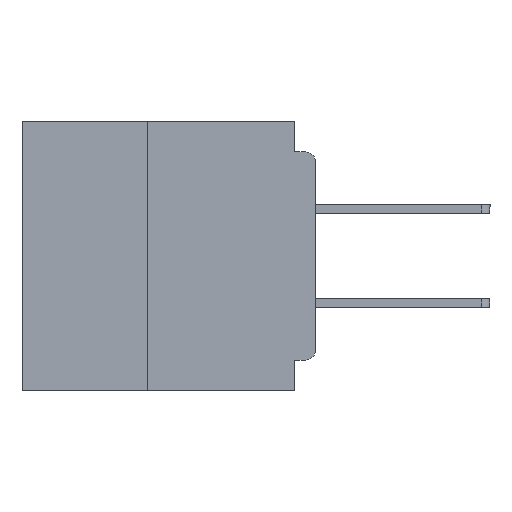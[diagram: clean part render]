
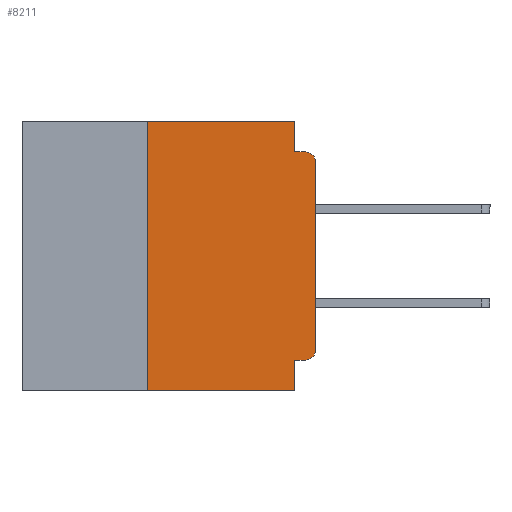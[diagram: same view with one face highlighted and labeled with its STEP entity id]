
A CAD part, left-side view. The second image highlights one B-rep face of the part: STEP entity #8211.
In plain terms, the highlighted planar face has unit normal (-1, 0, 0).
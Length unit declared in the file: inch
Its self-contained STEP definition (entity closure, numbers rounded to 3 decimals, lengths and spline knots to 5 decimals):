
#1073 = CARTESIAN_POINT ( 'NONE',  ( 0., 0., -0.34 ) ) ;
#1790 = CIRCLE ( 'NONE', #19528, 0.015 ) ;
#2159 = EDGE_CURVE ( 'NONE', #34190, #41145, #24736, .T. ) ;
#2250 = DIRECTION ( 'NONE',  ( 1., 0., 0. ) ) ;
#2364 = DIRECTION ( 'NONE',  ( 0., 0., -1. ) ) ;
#2720 = DIRECTION ( 'NONE',  ( 0., -1., 0. ) ) ;
#3563 = ORIENTED_EDGE ( 'NONE', *, *, #8190, .F. ) ;
#3602 = VERTEX_POINT ( 'NONE', #1073 ) ;
#4623 = CARTESIAN_POINT ( 'NONE',  ( 0., 0.015, -0.355 ) ) ;
#5570 = EDGE_CURVE ( 'NONE', #44614, #32273, #44536, .T. ) ;
#5735 = VECTOR ( 'NONE', #9948, 39.37008 ) ;
#6171 = CARTESIAN_POINT ( 'NONE',  ( 0., 0.437, 0. ) ) ;
#7149 = DIRECTION ( 'NONE',  ( 0., -1., 0. ) ) ;
#7772 = CARTESIAN_POINT ( 'NONE',  ( 0., 0., -0.355 ) ) ;
#8100 = EDGE_LOOP ( 'NONE', ( #29701, #22460, #29448, #16338, #37765, #3563, #18089, #26613, #38878, #15300 ) ) ;
#8190 = EDGE_CURVE ( 'NONE', #44614, #34190, #16019, .T. ) ;
#8211 = ADVANCED_FACE ( 'NONE', ( #45442 ), #40736, .F. ) ;
#9084 = VECTOR ( 'NONE', #38443, 39.37008 ) ;
#9948 = DIRECTION ( 'NONE',  ( 0., 0., 1. ) ) ;
#10064 = LINE ( 'NONE', #24833, #19144 ) ;
#10796 = EDGE_CURVE ( 'NONE', #41145, #42122, #39702, .T. ) ;
#10798 = AXIS2_PLACEMENT_3D ( 'NONE', #48417, #25735, #2364 ) ;
#11180 = DIRECTION ( 'NONE',  ( 0., 0., -1. ) ) ;
#11835 = VERTEX_POINT ( 'NONE', #25370 ) ;
#13703 = DIRECTION ( 'NONE',  ( 0., -1., 0. ) ) ;
#14224 = LINE ( 'NONE', #48257, #25846 ) ;
#14352 = VECTOR ( 'NONE', #2720, 39.37008 ) ;
#15084 = VECTOR ( 'NONE', #13703, 39.37008 ) ;
#15140 = CIRCLE ( 'NONE', #10798, 0.015 ) ;
#15300 = ORIENTED_EDGE ( 'NONE', *, *, #25182, .T. ) ;
#16019 = LINE ( 'NONE', #17402, #5735 ) ;
#16310 = EDGE_CURVE ( 'NONE', #42122, #11835, #26141, .T. ) ;
#16338 = ORIENTED_EDGE ( 'NONE', *, *, #10796, .F. ) ;
#17402 = CARTESIAN_POINT ( 'NONE',  ( 0., 0.25, -0.4 ) ) ;
#17687 = CARTESIAN_POINT ( 'NONE',  ( 0., 0.031, -0.045 ) ) ;
#18089 = ORIENTED_EDGE ( 'NONE', *, *, #5570, .T. ) ;
#19144 = VECTOR ( 'NONE', #21056, 39.37008 ) ;
#19262 = VECTOR ( 'NONE', #11180, 39.37008 ) ;
#19528 = AXIS2_PLACEMENT_3D ( 'NONE', #46022, #23209, #49741 ) ;
#21056 = DIRECTION ( 'NONE',  ( 0., 0., -1. ) ) ;
#21439 = VERTEX_POINT ( 'NONE', #39050 ) ;
#21489 = VERTEX_POINT ( 'NONE', #4623 ) ;
#22460 = ORIENTED_EDGE ( 'NONE', *, *, #35414, .T. ) ;
#22582 = CARTESIAN_POINT ( 'NONE',  ( 0., 0.25, -0.4 ) ) ;
#22644 = CARTESIAN_POINT ( 'NONE',  ( 0., 0., -0.06 ) ) ;
#23209 = DIRECTION ( 'NONE',  ( -1., 0., 0. ) ) ;
#24341 = CARTESIAN_POINT ( 'NONE',  ( 0., 0.031, -0.4 ) ) ;
#24736 = LINE ( 'NONE', #6171, #14352 ) ;
#24833 = CARTESIAN_POINT ( 'NONE',  ( 0., 0.031, -0.4 ) ) ;
#25182 = EDGE_CURVE ( 'NONE', #21489, #3602, #15140, .T. ) ;
#25370 = CARTESIAN_POINT ( 'NONE',  ( 0., 0.015, -0.045 ) ) ;
#25563 = DIRECTION ( 'NONE',  ( 0., 0., 1. ) ) ;
#25612 = CARTESIAN_POINT ( 'NONE',  ( 0., 0.437, 0. ) ) ;
#25735 = DIRECTION ( 'NONE',  ( -1., 0., 0. ) ) ;
#25846 = VECTOR ( 'NONE', #25563, 39.37008 ) ;
#26141 = LINE ( 'NONE', #38014, #45145 ) ;
#26613 = ORIENTED_EDGE ( 'NONE', *, *, #42640, .F. ) ;
#27244 = CARTESIAN_POINT ( 'NONE',  ( 0., 0.25, 0. ) ) ;
#29448 = ORIENTED_EDGE ( 'NONE', *, *, #16310, .F. ) ;
#29449 = DIRECTION ( 'NONE',  ( 0., 0., -1. ) ) ;
#29701 = ORIENTED_EDGE ( 'NONE', *, *, #39536, .T. ) ;
#30173 = VERTEX_POINT ( 'NONE', #22644 ) ;
#32273 = VERTEX_POINT ( 'NONE', #24341 ) ;
#34190 = VERTEX_POINT ( 'NONE', #27244 ) ;
#34305 = CARTESIAN_POINT ( 'NONE',  ( 0., 0.031, 0. ) ) ;
#35414 = EDGE_CURVE ( 'NONE', #30173, #11835, #1790, .T. ) ;
#36816 = CARTESIAN_POINT ( 'NONE',  ( 0., 0.437, -0.4 ) ) ;
#37765 = ORIENTED_EDGE ( 'NONE', *, *, #2159, .F. ) ;
#38014 = CARTESIAN_POINT ( 'NONE',  ( 0., 0., -0.045 ) ) ;
#38443 = DIRECTION ( 'NONE',  ( 0., 1., 0. ) ) ;
#38878 = ORIENTED_EDGE ( 'NONE', *, *, #40490, .F. ) ;
#38950 = AXIS2_PLACEMENT_3D ( 'NONE', #25612, #2250, #29449 ) ;
#39050 = CARTESIAN_POINT ( 'NONE',  ( 0., 0.031, -0.355 ) ) ;
#39536 = EDGE_CURVE ( 'NONE', #3602, #30173, #14224, .T. ) ;
#39702 = LINE ( 'NONE', #34305, #19262 ) ;
#40490 = EDGE_CURVE ( 'NONE', #21489, #21439, #49778, .T. ) ;
#40736 = PLANE ( 'NONE',  #38950 ) ;
#41145 = VERTEX_POINT ( 'NONE', #42665 ) ;
#42122 = VERTEX_POINT ( 'NONE', #17687 ) ;
#42640 = EDGE_CURVE ( 'NONE', #21439, #32273, #10064, .T. ) ;
#42665 = CARTESIAN_POINT ( 'NONE',  ( 0., 0.031, 0. ) ) ;
#44536 = LINE ( 'NONE', #36816, #15084 ) ;
#44614 = VERTEX_POINT ( 'NONE', #22582 ) ;
#45145 = VECTOR ( 'NONE', #7149, 39.37008 ) ;
#45442 = FACE_OUTER_BOUND ( 'NONE', #8100, .T. ) ;
#46022 = CARTESIAN_POINT ( 'NONE',  ( 0., 0.015, -0.06 ) ) ;
#48257 = CARTESIAN_POINT ( 'NONE',  ( 0., 0., 0. ) ) ;
#48417 = CARTESIAN_POINT ( 'NONE',  ( 0., 0.015, -0.34 ) ) ;
#49741 = DIRECTION ( 'NONE',  ( 0., 0., -1. ) ) ;
#49778 = LINE ( 'NONE', #7772, #9084 ) ;
